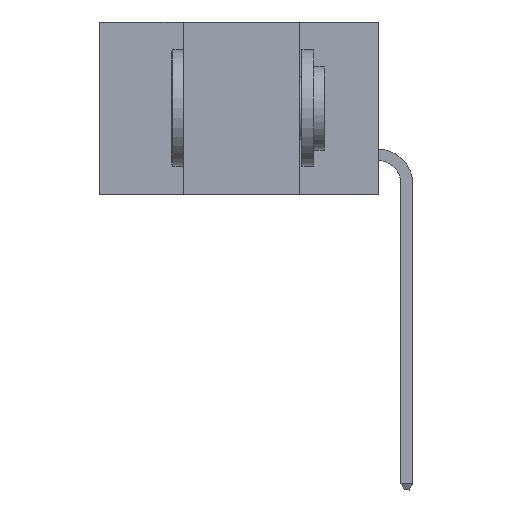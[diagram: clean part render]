
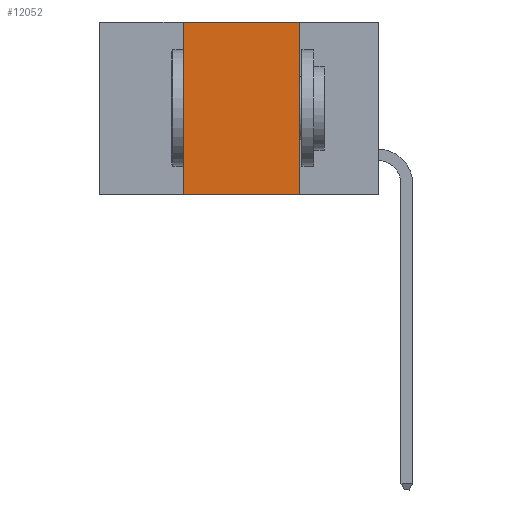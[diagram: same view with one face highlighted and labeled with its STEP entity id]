
A CAD part, left-side view. The second image highlights one B-rep face of the part: STEP entity #12052.
In plain terms, the highlighted planar face has unit normal (-1, 0, 0).
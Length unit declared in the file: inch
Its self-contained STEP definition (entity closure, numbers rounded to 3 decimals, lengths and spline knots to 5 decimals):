
#351 = FACE_OUTER_BOUND ( 'NONE', #19461, .T. ) ;
#1540 = ORIENTED_EDGE ( 'NONE', *, *, #18867, .T. ) ;
#1864 = CARTESIAN_POINT ( 'NONE',  ( 0., 0.17, 0. ) ) ;
#2282 = DIRECTION ( 'NONE',  ( 0., -1., 0. ) ) ;
#3264 = DIRECTION ( 'NONE',  ( 0., -1., 0. ) ) ;
#3484 = LINE ( 'NONE', #19614, #18910 ) ;
#4045 = CARTESIAN_POINT ( 'NONE',  ( 0., 0.6, 0. ) ) ;
#5734 = DIRECTION ( 'NONE',  ( 0., 0., -1. ) ) ;
#6170 = EDGE_CURVE ( 'NONE', #16800, #11872, #3484, .T. ) ;
#6374 = VERTEX_POINT ( 'NONE', #1864 ) ;
#6512 = VERTEX_POINT ( 'NONE', #12559 ) ;
#6658 = ORIENTED_EDGE ( 'NONE', *, *, #7631, .F. ) ;
#6729 = CARTESIAN_POINT ( 'NONE',  ( 0., 0.42, 0. ) ) ;
#7631 = EDGE_CURVE ( 'NONE', #6374, #6512, #14731, .T. ) ;
#8070 = CARTESIAN_POINT ( 'NONE',  ( 0., 0.6, -0.37 ) ) ;
#8158 = LINE ( 'NONE', #8070, #11543 ) ;
#8310 = CARTESIAN_POINT ( 'NONE',  ( 0., 0.42, -0.37 ) ) ;
#8404 = AXIS2_PLACEMENT_3D ( 'NONE', #19485, #19421, #5734 ) ;
#8969 = DIRECTION ( 'NONE',  ( 0., 0., 1. ) ) ;
#9765 = EDGE_CURVE ( 'NONE', #11872, #6374, #13409, .T. ) ;
#11543 = VECTOR ( 'NONE', #3264, 39.37008 ) ;
#11872 = VERTEX_POINT ( 'NONE', #6729 ) ;
#12052 = ADVANCED_FACE ( 'NONE', ( #351 ), #13166, .F. ) ;
#12514 = ORIENTED_EDGE ( 'NONE', *, *, #6170, .F. ) ;
#12559 = CARTESIAN_POINT ( 'NONE',  ( 0., 0.17, -0.37 ) ) ;
#12820 = ORIENTED_EDGE ( 'NONE', *, *, #9765, .F. ) ;
#13166 = PLANE ( 'NONE',  #8404 ) ;
#13169 = VECTOR ( 'NONE', #2282, 39.37008 ) ;
#13216 = DIRECTION ( 'NONE',  ( 0., 0., -1. ) ) ;
#13409 = LINE ( 'NONE', #4045, #13169 ) ;
#14236 = VECTOR ( 'NONE', #13216, 39.37008 ) ;
#14731 = LINE ( 'NONE', #16223, #14236 ) ;
#16223 = CARTESIAN_POINT ( 'NONE',  ( 0., 0.17, 0. ) ) ;
#16800 = VERTEX_POINT ( 'NONE', #8310 ) ;
#18867 = EDGE_CURVE ( 'NONE', #16800, #6512, #8158, .T. ) ;
#18910 = VECTOR ( 'NONE', #8969, 39.37008 ) ;
#19421 = DIRECTION ( 'NONE',  ( 1., 0., 0. ) ) ;
#19461 = EDGE_LOOP ( 'NONE', ( #6658, #12820, #12514, #1540 ) ) ;
#19485 = CARTESIAN_POINT ( 'NONE',  ( 0., 0.6, 0. ) ) ;
#19614 = CARTESIAN_POINT ( 'NONE',  ( 0., 0.42, 0. ) ) ;
